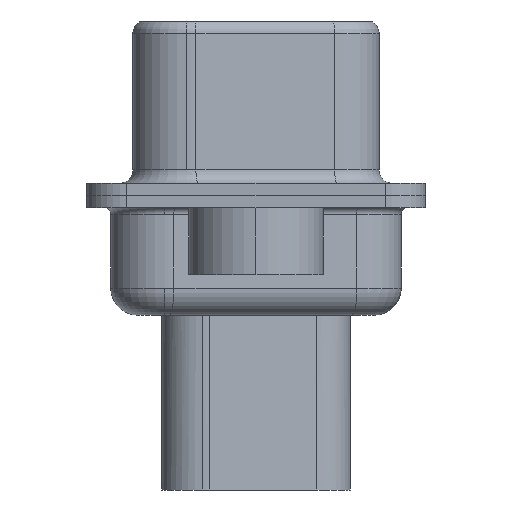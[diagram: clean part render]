
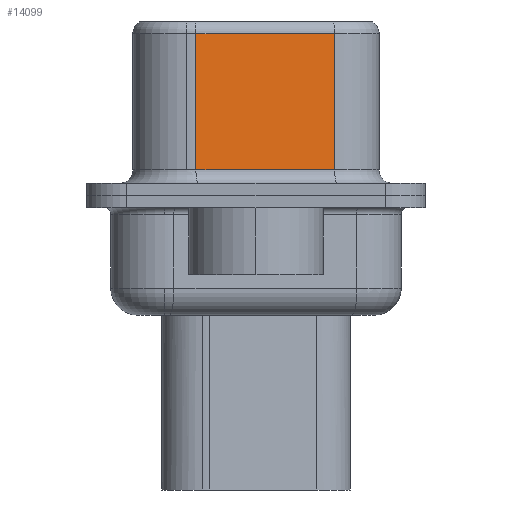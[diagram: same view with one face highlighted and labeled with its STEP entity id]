
A CAD part, left-side view. The second image highlights one B-rep face of the part: STEP entity #14099.
In plain terms, the highlighted planar face has unit normal (-0.985, -0.174, 0).
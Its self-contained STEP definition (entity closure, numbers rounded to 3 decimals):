
#580 = DIRECTION ( 'NONE',  ( 0., 0., -1. ) ) ;
#1793 = LINE ( 'NONE', #6301, #3832 ) ;
#1852 = CARTESIAN_POINT ( 'NONE',  ( 4.575, -2.927, 0.95 ) ) ;
#2388 = ORIENTED_EDGE ( 'NONE', *, *, #10385, .T. ) ;
#3022 = LINE ( 'NONE', #4128, #6655 ) ;
#3373 = VERTEX_POINT ( 'NONE', #1852 ) ;
#3455 = CARTESIAN_POINT ( 'NONE',  ( 4.575, -2.927, 6.02 ) ) ;
#3580 = FACE_OUTER_BOUND ( 'NONE', #8914, .T. ) ;
#3832 = VECTOR ( 'NONE', #14333, 1000. ) ;
#3858 = CARTESIAN_POINT ( 'NONE',  ( 4.575, -2.927, 6.02 ) ) ;
#4128 = CARTESIAN_POINT ( 'NONE',  ( 3.665, 2.233, 6.52 ) ) ;
#4343 = VERTEX_POINT ( 'NONE', #12548 ) ;
#4568 = DIRECTION ( 'NONE',  ( -0.174, 0.985, 0. ) ) ;
#4661 = DIRECTION ( 'NONE',  ( 0.174, -0.985, 0. ) ) ;
#4690 = PLANE ( 'NONE',  #6917 ) ;
#4841 = EDGE_CURVE ( 'NONE', #10135, #3373, #13724, .T. ) ;
#5954 = DIRECTION ( 'NONE',  ( 0.985, 0.174, 0. ) ) ;
#6144 = ORIENTED_EDGE ( 'NONE', *, *, #14515, .F. ) ;
#6301 = CARTESIAN_POINT ( 'NONE',  ( 4.575, -2.927, 6.52 ) ) ;
#6655 = VECTOR ( 'NONE', #580, 1000. ) ;
#6917 = AXIS2_PLACEMENT_3D ( 'NONE', #12642, #5954, #9308 ) ;
#7011 = LINE ( 'NONE', #3455, #8809 ) ;
#7127 = ORIENTED_EDGE ( 'NONE', *, *, #8400, .T. ) ;
#8400 = EDGE_CURVE ( 'NONE', #4343, #10135, #3022, .T. ) ;
#8809 = VECTOR ( 'NONE', #4568, 1000. ) ;
#8914 = EDGE_LOOP ( 'NONE', ( #6144, #2388, #7127, #10855 ) ) ;
#9308 = DIRECTION ( 'NONE',  ( -0.174, 0.985, 0. ) ) ;
#10135 = VERTEX_POINT ( 'NONE', #11933 ) ;
#10385 = EDGE_CURVE ( 'NONE', #10918, #4343, #7011, .T. ) ;
#10855 = ORIENTED_EDGE ( 'NONE', *, *, #4841, .T. ) ;
#10918 = VERTEX_POINT ( 'NONE', #3858 ) ;
#11933 = CARTESIAN_POINT ( 'NONE',  ( 3.665, 2.233, 0.95 ) ) ;
#12548 = CARTESIAN_POINT ( 'NONE',  ( 3.665, 2.233, 6.02 ) ) ;
#12642 = CARTESIAN_POINT ( 'NONE',  ( 4.575, -2.927, 6.52 ) ) ;
#13653 = CARTESIAN_POINT ( 'NONE',  ( 4.575, -2.927, 0.95 ) ) ;
#13724 = LINE ( 'NONE', #13653, #13871 ) ;
#13871 = VECTOR ( 'NONE', #4661, 1000. ) ;
#14099 = ADVANCED_FACE ( 'NONE', ( #3580 ), #4690, .F. ) ;
#14333 = DIRECTION ( 'NONE',  ( 0., 0., -1. ) ) ;
#14515 = EDGE_CURVE ( 'NONE', #10918, #3373, #1793, .T. ) ;
